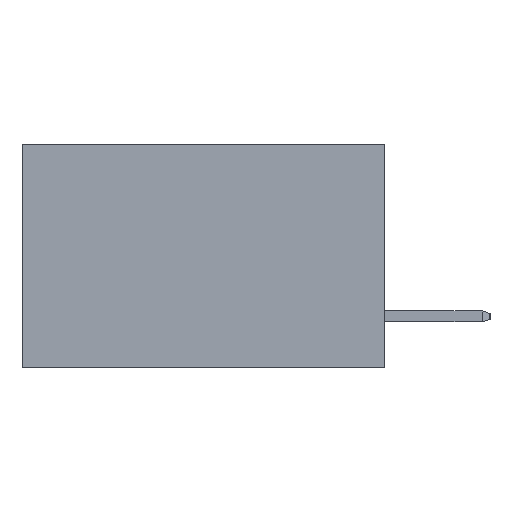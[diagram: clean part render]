
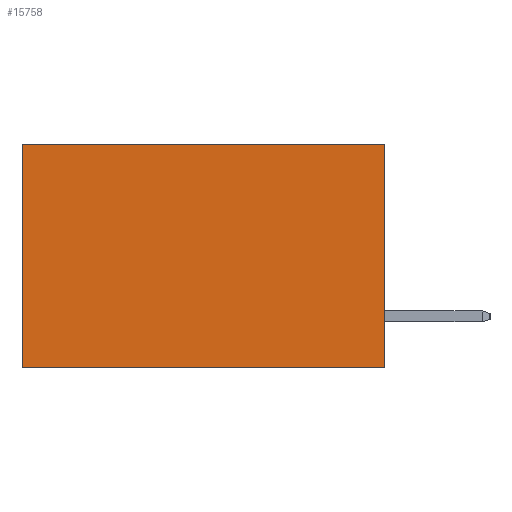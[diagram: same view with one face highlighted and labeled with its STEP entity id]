
A CAD part, left-side view. The second image highlights one B-rep face of the part: STEP entity #15758.
In plain terms, the highlighted planar face has unit normal (-1, 0, 0).
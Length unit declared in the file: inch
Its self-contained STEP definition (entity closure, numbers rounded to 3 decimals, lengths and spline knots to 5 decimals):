
#1528 = VERTEX_POINT ( 'NONE', #12399 ) ;
#1715 = EDGE_CURVE ( 'NONE', #4337, #10410, #4218, .T. ) ;
#3245 = VECTOR ( 'NONE', #18079, 39.37008 ) ;
#3565 = EDGE_CURVE ( 'NONE', #10410, #1528, #11213, .T. ) ;
#3724 = CARTESIAN_POINT ( 'NONE',  ( 0.2615, 0., -0.37 ) ) ;
#4218 = LINE ( 'NONE', #20188, #8151 ) ;
#4337 = VERTEX_POINT ( 'NONE', #19498 ) ;
#4488 = CARTESIAN_POINT ( 'NONE',  ( 0.2615, 0.6, 0. ) ) ;
#6376 = EDGE_LOOP ( 'NONE', ( #19575, #17908, #15443, #11904 ) ) ;
#8151 = VECTOR ( 'NONE', #19644, 39.37008 ) ;
#10283 = CARTESIAN_POINT ( 'NONE',  ( 0.2615, 0.6, -0.37 ) ) ;
#10410 = VERTEX_POINT ( 'NONE', #3724 ) ;
#11213 = LINE ( 'NONE', #17065, #16564 ) ;
#11904 = ORIENTED_EDGE ( 'NONE', *, *, #18865, .T. ) ;
#12399 = CARTESIAN_POINT ( 'NONE',  ( 0.2615, 0.6, -0.37 ) ) ;
#13154 = VERTEX_POINT ( 'NONE', #4488 ) ;
#13289 = EDGE_CURVE ( 'NONE', #13154, #1528, #18967, .T. ) ;
#13962 = AXIS2_PLACEMENT_3D ( 'NONE', #20005, #19555, #19464 ) ;
#15236 = DIRECTION ( 'NONE',  ( 0., 0., -1. ) ) ;
#15443 = ORIENTED_EDGE ( 'NONE', *, *, #1715, .F. ) ;
#15758 = ADVANCED_FACE ( 'NONE', ( #16657 ), #19903, .F. ) ;
#16564 = VECTOR ( 'NONE', #17359, 39.37008 ) ;
#16657 = FACE_OUTER_BOUND ( 'NONE', #6376, .T. ) ;
#17065 = CARTESIAN_POINT ( 'NONE',  ( 0.2615, 0., -0.37 ) ) ;
#17359 = DIRECTION ( 'NONE',  ( 0., 1., 0. ) ) ;
#17725 = CARTESIAN_POINT ( 'NONE',  ( 0.2615, 0., 0. ) ) ;
#17908 = ORIENTED_EDGE ( 'NONE', *, *, #3565, .F. ) ;
#18079 = DIRECTION ( 'NONE',  ( 0., 1., 0. ) ) ;
#18487 = VECTOR ( 'NONE', #15236, 39.37008 ) ;
#18865 = EDGE_CURVE ( 'NONE', #4337, #13154, #20079, .T. ) ;
#18967 = LINE ( 'NONE', #10283, #18487 ) ;
#19464 = DIRECTION ( 'NONE',  ( 0., 0., -1. ) ) ;
#19498 = CARTESIAN_POINT ( 'NONE',  ( 0.2615, 0., 0. ) ) ;
#19555 = DIRECTION ( 'NONE',  ( 1., 0., 0. ) ) ;
#19575 = ORIENTED_EDGE ( 'NONE', *, *, #13289, .T. ) ;
#19644 = DIRECTION ( 'NONE',  ( 0., 0., -1. ) ) ;
#19903 = PLANE ( 'NONE',  #13962 ) ;
#20005 = CARTESIAN_POINT ( 'NONE',  ( 0.2615, 0., -0.37 ) ) ;
#20079 = LINE ( 'NONE', #17725, #3245 ) ;
#20188 = CARTESIAN_POINT ( 'NONE',  ( 0.2615, 0., -0.37 ) ) ;
